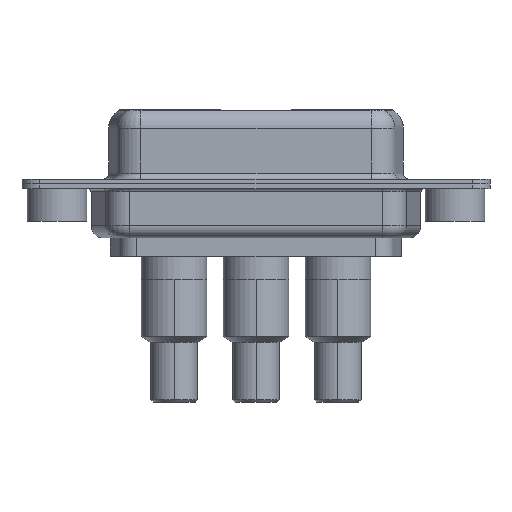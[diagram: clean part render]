
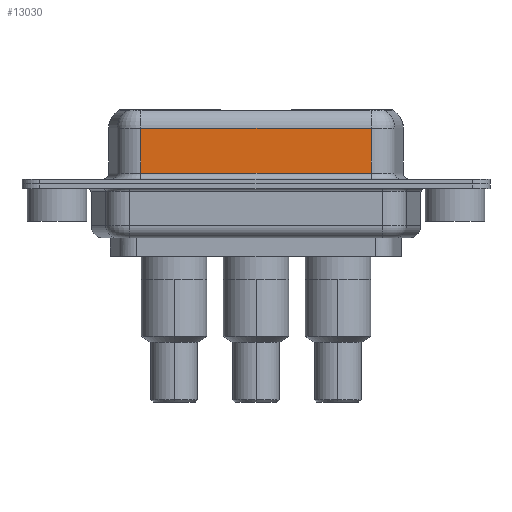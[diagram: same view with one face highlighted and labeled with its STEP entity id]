
A CAD part, front view. The second image highlights one B-rep face of the part: STEP entity #13030.
In plain terms, the highlighted planar face has unit normal (0, -1, 0).
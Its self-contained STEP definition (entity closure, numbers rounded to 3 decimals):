
#143 = LINE ( 'NONE', #2745, #2562 ) ;
#1211 = AXIS2_PLACEMENT_3D ( 'NONE', #8990, #10491, #1850 ) ;
#1850 = DIRECTION ( 'NONE',  ( 0., 0., 1. ) ) ;
#2282 = CARTESIAN_POINT ( 'NONE',  ( 26.287, -3.95, 4.65 ) ) ;
#2339 = ORIENTED_EDGE ( 'NONE', *, *, #9133, .T. ) ;
#2562 = VECTOR ( 'NONE', #5477, 1000. ) ;
#2745 = CARTESIAN_POINT ( 'NONE',  ( 7.013, -3.95, 6.4 ) ) ;
#4118 = VECTOR ( 'NONE', #9274, 1000. ) ;
#4801 = VERTEX_POINT ( 'NONE', #11817 ) ;
#4964 = EDGE_CURVE ( 'NONE', #4801, #13731, #9114, .T. ) ;
#5477 = DIRECTION ( 'NONE',  ( 0., 0., -1. ) ) ;
#5502 = FACE_OUTER_BOUND ( 'NONE', #7861, .T. ) ;
#5961 = ORIENTED_EDGE ( 'NONE', *, *, #4964, .T. ) ;
#6122 = EDGE_CURVE ( 'NONE', #9019, #4801, #143, .T. ) ;
#6386 = CARTESIAN_POINT ( 'NONE',  ( 26.287, -3.95, 6.4 ) ) ;
#7386 = EDGE_CURVE ( 'NONE', #8081, #13731, #7911, .T. ) ;
#7861 = EDGE_LOOP ( 'NONE', ( #7919, #2339, #14780, #5961 ) ) ;
#7911 = LINE ( 'NONE', #6386, #4118 ) ;
#7919 = ORIENTED_EDGE ( 'NONE', *, *, #7386, .F. ) ;
#8081 = VERTEX_POINT ( 'NONE', #2282 ) ;
#8414 = CARTESIAN_POINT ( 'NONE',  ( 26.287, -3.95, 4.65 ) ) ;
#8929 = PLANE ( 'NONE',  #1211 ) ;
#8976 = VECTOR ( 'NONE', #17272, 1000. ) ;
#8990 = CARTESIAN_POINT ( 'NONE',  ( 26.287, -3.95, 6.4 ) ) ;
#9019 = VERTEX_POINT ( 'NONE', #17035 ) ;
#9114 = LINE ( 'NONE', #15591, #16580 ) ;
#9133 = EDGE_CURVE ( 'NONE', #8081, #9019, #11987, .T. ) ;
#9274 = DIRECTION ( 'NONE',  ( 0., 0., -1. ) ) ;
#10491 = DIRECTION ( 'NONE',  ( 0., 1., 0. ) ) ;
#11817 = CARTESIAN_POINT ( 'NONE',  ( 7.013, -3.95, 0.9 ) ) ;
#11987 = LINE ( 'NONE', #8414, #8976 ) ;
#13030 = ADVANCED_FACE ( 'NONE', ( #5502 ), #8929, .F. ) ;
#13731 = VERTEX_POINT ( 'NONE', #16997 ) ;
#14780 = ORIENTED_EDGE ( 'NONE', *, *, #6122, .T. ) ;
#15591 = CARTESIAN_POINT ( 'NONE',  ( 26.287, -3.95, 0.9 ) ) ;
#16098 = DIRECTION ( 'NONE',  ( 1., 0., 0. ) ) ;
#16580 = VECTOR ( 'NONE', #16098, 1000. ) ;
#16997 = CARTESIAN_POINT ( 'NONE',  ( 26.287, -3.95, 0.9 ) ) ;
#17035 = CARTESIAN_POINT ( 'NONE',  ( 7.013, -3.95, 4.65 ) ) ;
#17272 = DIRECTION ( 'NONE',  ( -1., 0., 0. ) ) ;
